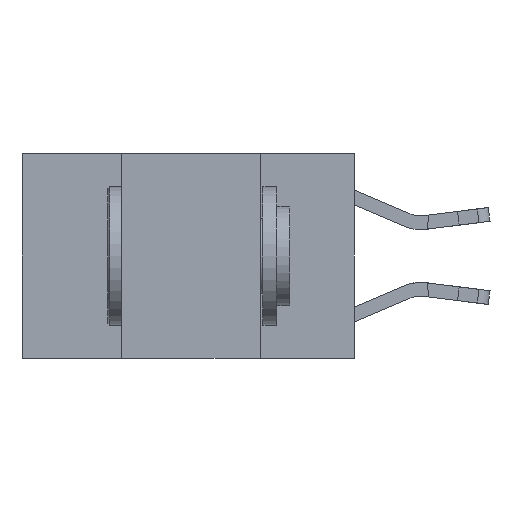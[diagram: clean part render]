
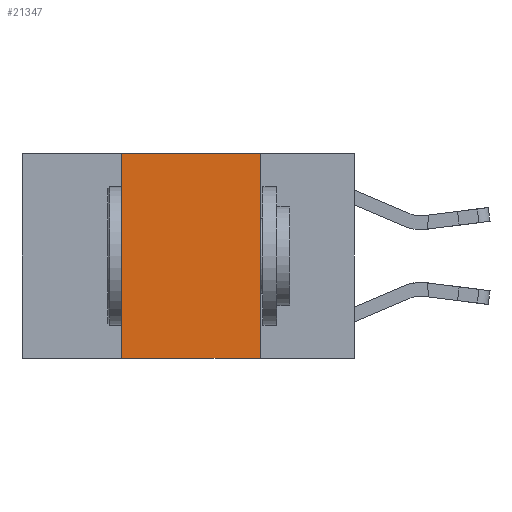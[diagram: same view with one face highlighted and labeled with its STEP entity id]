
A CAD part, left-side view. The second image highlights one B-rep face of the part: STEP entity #21347.
In plain terms, the highlighted planar face has unit normal (-1, 0, 0).
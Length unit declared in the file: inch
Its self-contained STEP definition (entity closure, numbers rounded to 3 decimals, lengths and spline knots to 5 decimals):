
#1543 = DIRECTION ( 'NONE',  ( 0., 0., -1. ) ) ;
#3737 = VERTEX_POINT ( 'NONE', #13347 ) ;
#3987 = VERTEX_POINT ( 'NONE', #23805 ) ;
#4948 = LINE ( 'NONE', #11354, #8391 ) ;
#5560 = FACE_OUTER_BOUND ( 'NONE', #19778, .T. ) ;
#5998 = PLANE ( 'NONE',  #26684 ) ;
#8215 = EDGE_CURVE ( 'NONE', #23750, #3737, #9320, .T. ) ;
#8391 = VECTOR ( 'NONE', #14063, 39.37008 ) ;
#8906 = ORIENTED_EDGE ( 'NONE', *, *, #26754, .F. ) ;
#9217 = DIRECTION ( 'NONE',  ( 0., 0., 1. ) ) ;
#9320 = LINE ( 'NONE', #18449, #22191 ) ;
#10751 = DIRECTION ( 'NONE',  ( 1., 0., 0. ) ) ;
#11354 = CARTESIAN_POINT ( 'NONE',  ( 0., 0.6, -0.37 ) ) ;
#11605 = CARTESIAN_POINT ( 'NONE',  ( 0., 0.42, 0. ) ) ;
#11610 = EDGE_CURVE ( 'NONE', #24788, #3987, #4948, .T. ) ;
#12620 = CARTESIAN_POINT ( 'NONE',  ( 0., 0.17, 0. ) ) ;
#13347 = CARTESIAN_POINT ( 'NONE',  ( 0., 0.17, 0. ) ) ;
#14063 = DIRECTION ( 'NONE',  ( 0., -1., 0. ) ) ;
#18449 = CARTESIAN_POINT ( 'NONE',  ( 0., 0.6, 0. ) ) ;
#19349 = LINE ( 'NONE', #12620, #29256 ) ;
#19778 = EDGE_LOOP ( 'NONE', ( #27429, #23530, #8906, #26080 ) ) ;
#21347 = ADVANCED_FACE ( 'NONE', ( #5560 ), #5998, .F. ) ;
#21588 = VECTOR ( 'NONE', #9217, 39.37008 ) ;
#21762 = CARTESIAN_POINT ( 'NONE',  ( 0., 0.42, 0. ) ) ;
#21970 = CARTESIAN_POINT ( 'NONE',  ( 0., 0.6, 0. ) ) ;
#22191 = VECTOR ( 'NONE', #25626, 39.37008 ) ;
#23423 = LINE ( 'NONE', #11605, #21588 ) ;
#23530 = ORIENTED_EDGE ( 'NONE', *, *, #8215, .F. ) ;
#23750 = VERTEX_POINT ( 'NONE', #21762 ) ;
#23805 = CARTESIAN_POINT ( 'NONE',  ( 0., 0.17, -0.37 ) ) ;
#24788 = VERTEX_POINT ( 'NONE', #26497 ) ;
#25626 = DIRECTION ( 'NONE',  ( 0., -1., 0. ) ) ;
#26080 = ORIENTED_EDGE ( 'NONE', *, *, #11610, .T. ) ;
#26497 = CARTESIAN_POINT ( 'NONE',  ( 0., 0.42, -0.37 ) ) ;
#26684 = AXIS2_PLACEMENT_3D ( 'NONE', #21970, #10751, #1543 ) ;
#26754 = EDGE_CURVE ( 'NONE', #24788, #23750, #23423, .T. ) ;
#27323 = EDGE_CURVE ( 'NONE', #3737, #3987, #19349, .T. ) ;
#27429 = ORIENTED_EDGE ( 'NONE', *, *, #27323, .F. ) ;
#28480 = DIRECTION ( 'NONE',  ( 0., 0., -1. ) ) ;
#29256 = VECTOR ( 'NONE', #28480, 39.37008 ) ;
